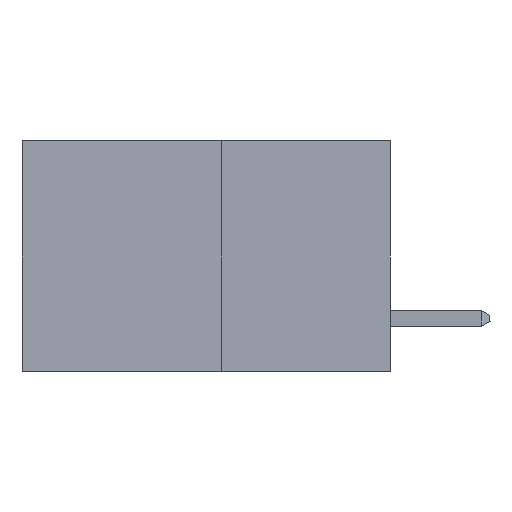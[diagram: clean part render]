
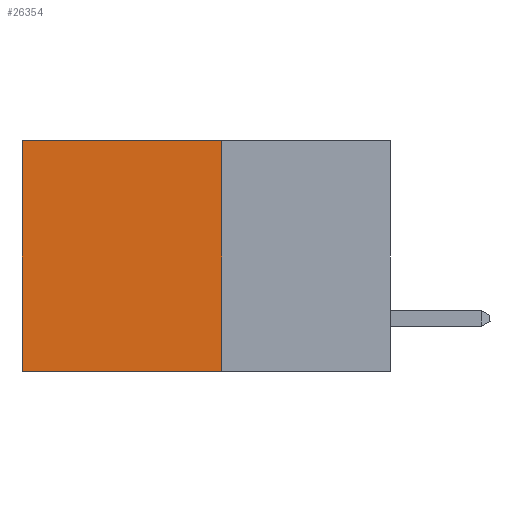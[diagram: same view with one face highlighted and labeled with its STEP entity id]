
A CAD part, left-side view. The second image highlights one B-rep face of the part: STEP entity #26354.
In plain terms, the highlighted planar face has unit normal (-1, 0, 0).
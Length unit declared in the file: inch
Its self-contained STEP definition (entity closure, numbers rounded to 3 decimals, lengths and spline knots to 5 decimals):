
#228 = CARTESIAN_POINT ( 'NONE',  ( 0.277, 0.59, -0.37 ) ) ;
#971 = LINE ( 'NONE', #27583, #13207 ) ;
#2810 = VECTOR ( 'NONE', #17836, 39.37008 ) ;
#2911 = CARTESIAN_POINT ( 'NONE',  ( 0.277, 0.27, 0. ) ) ;
#4552 = LINE ( 'NONE', #7654, #28800 ) ;
#5609 = VERTEX_POINT ( 'NONE', #27500 ) ;
#7654 = CARTESIAN_POINT ( 'NONE',  ( 0.277, 0.27, -0.37 ) ) ;
#10444 = VERTEX_POINT ( 'NONE', #27841 ) ;
#11100 = LINE ( 'NONE', #228, #30300 ) ;
#12562 = VERTEX_POINT ( 'NONE', #2911 ) ;
#13207 = VECTOR ( 'NONE', #29992, 39.37008 ) ;
#13849 = CARTESIAN_POINT ( 'NONE',  ( 0.277, 0.27, -0.37 ) ) ;
#14861 = DIRECTION ( 'NONE',  ( 0., 0., -1. ) ) ;
#14868 = AXIS2_PLACEMENT_3D ( 'NONE', #13849, #30634, #16264 ) ;
#15427 = CARTESIAN_POINT ( 'NONE',  ( 0.277, 0.27, 0. ) ) ;
#16264 = DIRECTION ( 'NONE',  ( 0., 0., -1. ) ) ;
#16539 = LINE ( 'NONE', #15427, #2810 ) ;
#17267 = DIRECTION ( 'NONE',  ( 0., 1., 0. ) ) ;
#17836 = DIRECTION ( 'NONE',  ( 0., 1., 0. ) ) ;
#22635 = ORIENTED_EDGE ( 'NONE', *, *, #23765, .F. ) ;
#22776 = FACE_OUTER_BOUND ( 'NONE', #25863, .T. ) ;
#23362 = CARTESIAN_POINT ( 'NONE',  ( 0.277, 0.27, -0.37 ) ) ;
#23731 = ORIENTED_EDGE ( 'NONE', *, *, #28991, .F. ) ;
#23765 = EDGE_CURVE ( 'NONE', #12562, #27056, #971, .T. ) ;
#24263 = EDGE_CURVE ( 'NONE', #12562, #10444, #16539, .T. ) ;
#25809 = PLANE ( 'NONE',  #14868 ) ;
#25863 = EDGE_LOOP ( 'NONE', ( #28970, #23731, #22635, #30997 ) ) ;
#26354 = ADVANCED_FACE ( 'NONE', ( #22776 ), #25809, .F. ) ;
#27056 = VERTEX_POINT ( 'NONE', #23362 ) ;
#27500 = CARTESIAN_POINT ( 'NONE',  ( 0.277, 0.59, -0.37 ) ) ;
#27583 = CARTESIAN_POINT ( 'NONE',  ( 0.277, 0.27, -0.37 ) ) ;
#27841 = CARTESIAN_POINT ( 'NONE',  ( 0.277, 0.59, 0. ) ) ;
#28800 = VECTOR ( 'NONE', #17267, 39.37008 ) ;
#28945 = EDGE_CURVE ( 'NONE', #10444, #5609, #11100, .T. ) ;
#28970 = ORIENTED_EDGE ( 'NONE', *, *, #28945, .T. ) ;
#28991 = EDGE_CURVE ( 'NONE', #27056, #5609, #4552, .T. ) ;
#29992 = DIRECTION ( 'NONE',  ( 0., 0., -1. ) ) ;
#30300 = VECTOR ( 'NONE', #14861, 39.37008 ) ;
#30634 = DIRECTION ( 'NONE',  ( 1., 0., 0. ) ) ;
#30997 = ORIENTED_EDGE ( 'NONE', *, *, #24263, .T. ) ;
